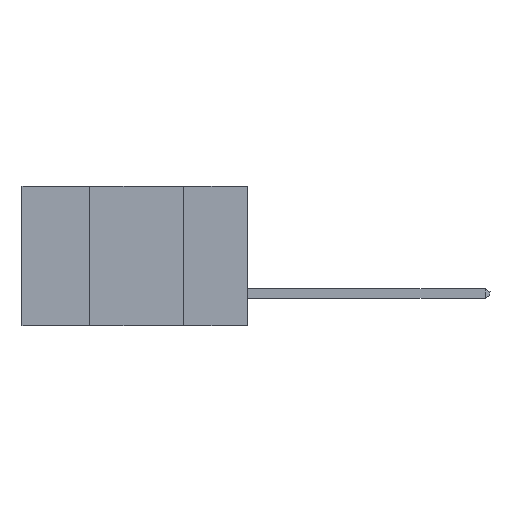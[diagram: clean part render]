
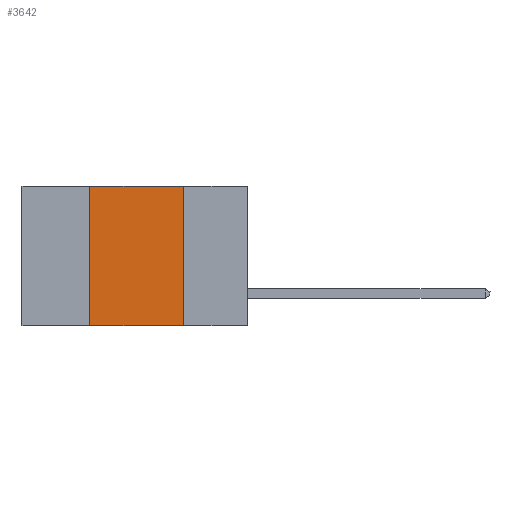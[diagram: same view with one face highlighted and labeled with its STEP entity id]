
A CAD part, left-side view. The second image highlights one B-rep face of the part: STEP entity #3642.
In plain terms, the highlighted planar face has unit normal (-1, 0, 0).
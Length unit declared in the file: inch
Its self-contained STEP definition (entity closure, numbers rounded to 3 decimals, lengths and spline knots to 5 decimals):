
#178 = VECTOR ( 'NONE', #4765, 39.37008 ) ;
#915 = EDGE_CURVE ( 'NONE', #4771, #5408, #5048, .T. ) ;
#1224 = VECTOR ( 'NONE', #8435, 39.37008 ) ;
#1349 = DIRECTION ( 'NONE',  ( 1., 0., 0. ) ) ;
#1863 = EDGE_LOOP ( 'NONE', ( #8020, #3406, #3912, #4312 ) ) ;
#1888 = DIRECTION ( 'NONE',  ( 0., -1., 0. ) ) ;
#2039 = AXIS2_PLACEMENT_3D ( 'NONE', #6164, #1349, #6761 ) ;
#2299 = VERTEX_POINT ( 'NONE', #7358 ) ;
#2626 = EDGE_CURVE ( 'NONE', #5408, #2861, #4350, .T. ) ;
#2861 = VERTEX_POINT ( 'NONE', #4229 ) ;
#3034 = CARTESIAN_POINT ( 'NONE',  ( 0., 0.17, 0. ) ) ;
#3406 = ORIENTED_EDGE ( 'NONE', *, *, #915, .F. ) ;
#3642 = ADVANCED_FACE ( 'NONE', ( #8221 ), #7404, .F. ) ;
#3912 = ORIENTED_EDGE ( 'NONE', *, *, #4634, .F. ) ;
#4229 = CARTESIAN_POINT ( 'NONE',  ( 0., 0.17, -0.37 ) ) ;
#4312 = ORIENTED_EDGE ( 'NONE', *, *, #4523, .T. ) ;
#4345 = DIRECTION ( 'NONE',  ( 0., -1., 0. ) ) ;
#4350 = LINE ( 'NONE', #5641, #1224 ) ;
#4523 = EDGE_CURVE ( 'NONE', #2299, #2861, #8119, .T. ) ;
#4634 = EDGE_CURVE ( 'NONE', #2299, #4771, #7689, .T. ) ;
#4765 = DIRECTION ( 'NONE',  ( 0., 0., 1. ) ) ;
#4771 = VERTEX_POINT ( 'NONE', #6578 ) ;
#5048 = LINE ( 'NONE', #7830, #8676 ) ;
#5408 = VERTEX_POINT ( 'NONE', #3034 ) ;
#5641 = CARTESIAN_POINT ( 'NONE',  ( 0., 0.17, -0.37 ) ) ;
#6164 = CARTESIAN_POINT ( 'NONE',  ( 0., 0.6, 0. ) ) ;
#6578 = CARTESIAN_POINT ( 'NONE',  ( 0., 0.42, 0. ) ) ;
#6761 = DIRECTION ( 'NONE',  ( 0., 0., -1. ) ) ;
#6819 = CARTESIAN_POINT ( 'NONE',  ( 0., 0.6, -0.37 ) ) ;
#6867 = CARTESIAN_POINT ( 'NONE',  ( 0., 0.42, -0.37 ) ) ;
#7139 = VECTOR ( 'NONE', #1888, 39.37008 ) ;
#7358 = CARTESIAN_POINT ( 'NONE',  ( 0., 0.42, -0.37 ) ) ;
#7404 = PLANE ( 'NONE',  #2039 ) ;
#7689 = LINE ( 'NONE', #6867, #178 ) ;
#7830 = CARTESIAN_POINT ( 'NONE',  ( 0., 0.6, 0. ) ) ;
#8020 = ORIENTED_EDGE ( 'NONE', *, *, #2626, .F. ) ;
#8119 = LINE ( 'NONE', #6819, #7139 ) ;
#8221 = FACE_OUTER_BOUND ( 'NONE', #1863, .T. ) ;
#8435 = DIRECTION ( 'NONE',  ( 0., 0., -1. ) ) ;
#8676 = VECTOR ( 'NONE', #4345, 39.37008 ) ;
